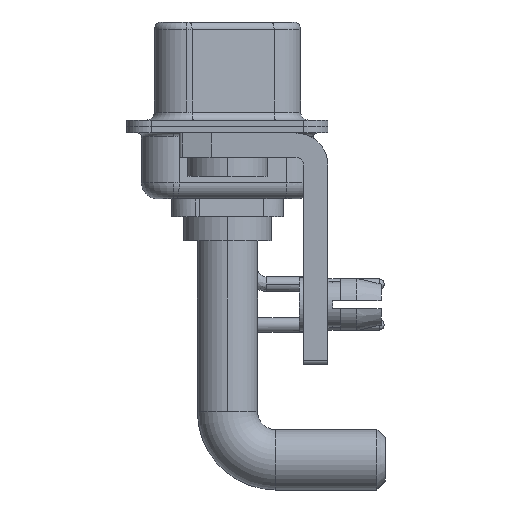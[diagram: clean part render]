
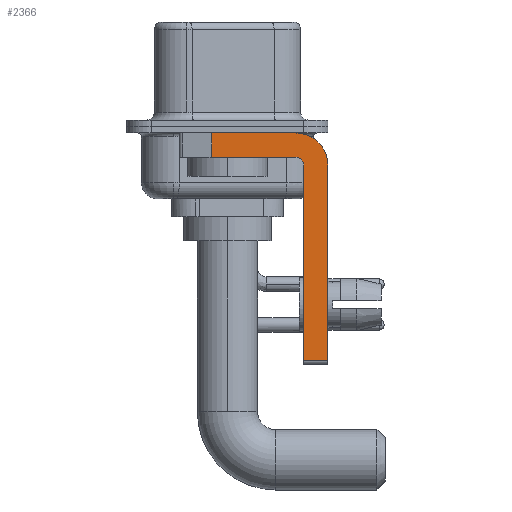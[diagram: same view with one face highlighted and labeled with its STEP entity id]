
A CAD part, left-side view. The second image highlights one B-rep face of the part: STEP entity #2366.
In plain terms, the highlighted planar face has unit normal (-1, 0, 0).
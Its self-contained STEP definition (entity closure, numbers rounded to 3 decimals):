
#394 = CARTESIAN_POINT ( 'NONE',  ( -2.9, -4.25, -2.4 ) ) ;
#1035 = VERTEX_POINT ( 'NONE', #9701 ) ;
#1907 = DIRECTION ( 'NONE',  ( 0., -1., 0. ) ) ;
#2366 = ADVANCED_FACE ( 'NONE', ( #16520 ), #3542, .F. ) ;
#3250 = DIRECTION ( 'NONE',  ( 1., 0., 0. ) ) ;
#3396 = CARTESIAN_POINT ( 'NONE',  ( -2.9, 3., -0.4 ) ) ;
#3542 = PLANE ( 'NONE',  #11781 ) ;
#3828 = DIRECTION ( 'NONE',  ( 0., 0., -1. ) ) ;
#4312 = ORIENTED_EDGE ( 'NONE', *, *, #16261, .F. ) ;
#4433 = EDGE_CURVE ( 'NONE', #4469, #5684, #5477, .T. ) ;
#4469 = VERTEX_POINT ( 'NONE', #14651 ) ;
#4636 = VECTOR ( 'NONE', #1907, 1000. ) ;
#4783 = EDGE_CURVE ( 'NONE', #26498, #1035, #5898, .T. ) ;
#5201 = ORIENTED_EDGE ( 'NONE', *, *, #26304, .F. ) ;
#5477 = CIRCLE ( 'NONE', #21414, 2. ) ;
#5679 = DIRECTION ( 'NONE',  ( 0., 0., -1. ) ) ;
#5684 = VERTEX_POINT ( 'NONE', #14301 ) ;
#5898 = CIRCLE ( 'NONE', #21838, 0.5 ) ;
#6116 = CARTESIAN_POINT ( 'NONE',  ( -2.9, 0.978, -1.9 ) ) ;
#6388 = CARTESIAN_POINT ( 'NONE',  ( -2.9, -6.25, -14.55 ) ) ;
#7155 = ORIENTED_EDGE ( 'NONE', *, *, #18512, .T. ) ;
#7301 = LINE ( 'NONE', #22988, #24856 ) ;
#7607 = DIRECTION ( 'NONE',  ( 0., 0., 1. ) ) ;
#7657 = VERTEX_POINT ( 'NONE', #6116 ) ;
#9199 = LINE ( 'NONE', #17896, #13364 ) ;
#9701 = CARTESIAN_POINT ( 'NONE',  ( -2.9, -4.25, -1.9 ) ) ;
#10115 = LINE ( 'NONE', #18815, #17927 ) ;
#10869 = CARTESIAN_POINT ( 'NONE',  ( -2.9, -4.25, -14.55 ) ) ;
#11781 = AXIS2_PLACEMENT_3D ( 'NONE', #12244, #21074, #18799 ) ;
#11953 = DIRECTION ( 'NONE',  ( 0., -1., 0. ) ) ;
#12244 = CARTESIAN_POINT ( 'NONE',  ( -2.9, -4.25, -2.4 ) ) ;
#12368 = CARTESIAN_POINT ( 'NONE',  ( -2.9, -4.25, -2.4 ) ) ;
#13364 = VECTOR ( 'NONE', #26608, 1000. ) ;
#13548 = VERTEX_POINT ( 'NONE', #16591 ) ;
#13563 = EDGE_CURVE ( 'NONE', #13548, #26498, #27013, .T. ) ;
#13616 = ORIENTED_EDGE ( 'NONE', *, *, #13563, .F. ) ;
#13634 = DIRECTION ( 'NONE',  ( 0., 0., 1. ) ) ;
#14277 = DIRECTION ( 'NONE',  ( 0., 0., -1. ) ) ;
#14301 = CARTESIAN_POINT ( 'NONE',  ( -2.9, -6.25, -2.4 ) ) ;
#14651 = CARTESIAN_POINT ( 'NONE',  ( -2.9, -4.25, -0.4 ) ) ;
#15024 = EDGE_CURVE ( 'NONE', #13548, #27812, #19295, .T. ) ;
#15502 = VERTEX_POINT ( 'NONE', #21541 ) ;
#15618 = CARTESIAN_POINT ( 'NONE',  ( -2.9, -4.75, -2.4 ) ) ;
#16187 = VECTOR ( 'NONE', #11953, 1000. ) ;
#16261 = EDGE_CURVE ( 'NONE', #1035, #7657, #9199, .T. ) ;
#16429 = VECTOR ( 'NONE', #7607, 1000. ) ;
#16520 = FACE_OUTER_BOUND ( 'NONE', #27525, .T. ) ;
#16591 = CARTESIAN_POINT ( 'NONE',  ( -2.9, -4.75, -14.55 ) ) ;
#16642 = ORIENTED_EDGE ( 'NONE', *, *, #27694, .F. ) ;
#17896 = CARTESIAN_POINT ( 'NONE',  ( -2.9, -4.25, -1.9 ) ) ;
#17927 = VECTOR ( 'NONE', #3828, 1000. ) ;
#18299 = CARTESIAN_POINT ( 'NONE',  ( -2.9, -4.75, -14.8 ) ) ;
#18512 = EDGE_CURVE ( 'NONE', #15502, #7657, #10115, .T. ) ;
#18799 = DIRECTION ( 'NONE',  ( 0., 0., -1. ) ) ;
#18815 = CARTESIAN_POINT ( 'NONE',  ( -2.9, 0.978, -1.9 ) ) ;
#19295 = LINE ( 'NONE', #10869, #4636 ) ;
#21074 = DIRECTION ( 'NONE',  ( 1., 0., 0. ) ) ;
#21414 = AXIS2_PLACEMENT_3D ( 'NONE', #12368, #3250, #5679 ) ;
#21541 = CARTESIAN_POINT ( 'NONE',  ( -2.9, 0.978, -0.4 ) ) ;
#21838 = AXIS2_PLACEMENT_3D ( 'NONE', #394, #22472, #13634 ) ;
#22472 = DIRECTION ( 'NONE',  ( -1., 0., 0. ) ) ;
#22795 = ORIENTED_EDGE ( 'NONE', *, *, #4783, .F. ) ;
#22805 = ORIENTED_EDGE ( 'NONE', *, *, #15024, .T. ) ;
#22988 = CARTESIAN_POINT ( 'NONE',  ( -2.9, -6.25, -2.4 ) ) ;
#23088 = LINE ( 'NONE', #3396, #16187 ) ;
#24856 = VECTOR ( 'NONE', #14277, 1000. ) ;
#26304 = EDGE_CURVE ( 'NONE', #15502, #4469, #23088, .T. ) ;
#26498 = VERTEX_POINT ( 'NONE', #15618 ) ;
#26608 = DIRECTION ( 'NONE',  ( 0., 1., 0. ) ) ;
#26919 = ORIENTED_EDGE ( 'NONE', *, *, #4433, .F. ) ;
#27013 = LINE ( 'NONE', #18299, #16429 ) ;
#27525 = EDGE_LOOP ( 'NONE', ( #5201, #7155, #4312, #22795, #13616, #22805, #16642, #26919 ) ) ;
#27694 = EDGE_CURVE ( 'NONE', #5684, #27812, #7301, .T. ) ;
#27812 = VERTEX_POINT ( 'NONE', #6388 ) ;
